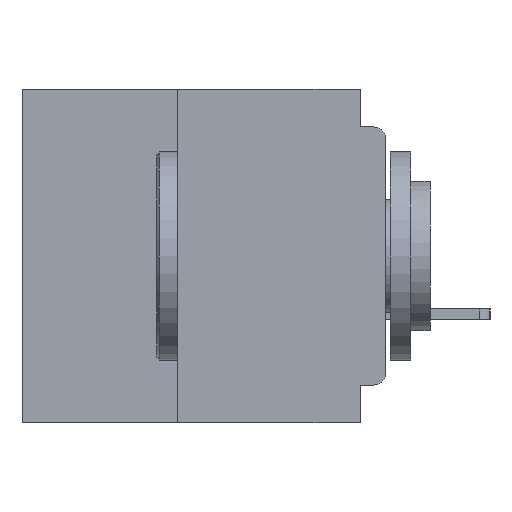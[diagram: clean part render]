
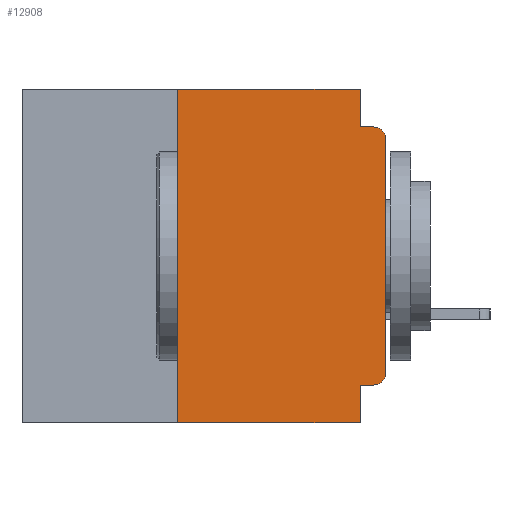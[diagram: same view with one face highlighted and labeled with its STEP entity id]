
A CAD part, left-side view. The second image highlights one B-rep face of the part: STEP entity #12908.
In plain terms, the highlighted planar face has unit normal (-1, 0, 0).
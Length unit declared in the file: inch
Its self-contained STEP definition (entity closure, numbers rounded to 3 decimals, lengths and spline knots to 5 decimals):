
#207 = LINE ( 'NONE', #11736, #41279 ) ;
#290 = VECTOR ( 'NONE', #2912, 39.37008 ) ;
#741 = VERTEX_POINT ( 'NONE', #13909 ) ;
#750 = DIRECTION ( 'NONE',  ( 0., 0., -1. ) ) ;
#1544 = LINE ( 'NONE', #10858, #290 ) ;
#1704 = EDGE_CURVE ( 'NONE', #27316, #12197, #5663, .T. ) ;
#1719 = ORIENTED_EDGE ( 'NONE', *, *, #18639, .F. ) ;
#1902 = VERTEX_POINT ( 'NONE', #48095 ) ;
#2888 = VERTEX_POINT ( 'NONE', #45726 ) ;
#2912 = DIRECTION ( 'NONE',  ( 0., 1., 0. ) ) ;
#3446 = LINE ( 'NONE', #10062, #22133 ) ;
#4412 = VECTOR ( 'NONE', #18042, 39.37008 ) ;
#4454 = EDGE_CURVE ( 'NONE', #5915, #27316, #51467, .T. ) ;
#4998 = DIRECTION ( 'NONE',  ( 0., 0., -1. ) ) ;
#5009 = CARTESIAN_POINT ( 'NONE',  ( 0., 0.437, -0.4 ) ) ;
#5066 = DIRECTION ( 'NONE',  ( -1., 0., 0. ) ) ;
#5075 = CARTESIAN_POINT ( 'NONE',  ( 0., 0.015, -0.34 ) ) ;
#5244 = PLANE ( 'NONE',  #33395 ) ;
#5475 = ORIENTED_EDGE ( 'NONE', *, *, #14504, .F. ) ;
#5663 = LINE ( 'NONE', #18956, #4412 ) ;
#5915 = VERTEX_POINT ( 'NONE', #47709 ) ;
#6281 = DIRECTION ( 'NONE',  ( 0., -1., 0. ) ) ;
#6307 = VECTOR ( 'NONE', #750, 39.37008 ) ;
#6487 = VERTEX_POINT ( 'NONE', #47653 ) ;
#6509 = DIRECTION ( 'NONE',  ( 0., -1., 0. ) ) ;
#9202 = DIRECTION ( 'NONE',  ( 0., 0., -1. ) ) ;
#10062 = CARTESIAN_POINT ( 'NONE',  ( 0., 0., -0.045 ) ) ;
#10858 = CARTESIAN_POINT ( 'NONE',  ( 0., 0., -0.355 ) ) ;
#11176 = CARTESIAN_POINT ( 'NONE',  ( 0., 0.015, -0.06 ) ) ;
#11736 = CARTESIAN_POINT ( 'NONE',  ( 0., 0.031, 0. ) ) ;
#12105 = EDGE_CURVE ( 'NONE', #12197, #18398, #21471, .T. ) ;
#12197 = VERTEX_POINT ( 'NONE', #19746 ) ;
#12536 = CARTESIAN_POINT ( 'NONE',  ( 0., 0.015, -0.045 ) ) ;
#12908 = ADVANCED_FACE ( 'NONE', ( #34014 ), #5244, .F. ) ;
#13524 = ORIENTED_EDGE ( 'NONE', *, *, #14053, .F. ) ;
#13909 = CARTESIAN_POINT ( 'NONE',  ( 0., 0.031, -0.4 ) ) ;
#14053 = EDGE_CURVE ( 'NONE', #14677, #2888, #207, .T. ) ;
#14504 = EDGE_CURVE ( 'NONE', #43937, #14677, #30729, .T. ) ;
#14677 = VERTEX_POINT ( 'NONE', #43330 ) ;
#15201 = DIRECTION ( 'NONE',  ( 0., 0., -1. ) ) ;
#15613 = LINE ( 'NONE', #24624, #6307 ) ;
#17323 = ORIENTED_EDGE ( 'NONE', *, *, #47789, .T. ) ;
#18042 = DIRECTION ( 'NONE',  ( 0., 0., 1. ) ) ;
#18398 = VERTEX_POINT ( 'NONE', #12536 ) ;
#18639 = EDGE_CURVE ( 'NONE', #2888, #18398, #3446, .T. ) ;
#18956 = CARTESIAN_POINT ( 'NONE',  ( 0., 0., 0. ) ) ;
#19148 = ORIENTED_EDGE ( 'NONE', *, *, #1704, .T. ) ;
#19537 = EDGE_CURVE ( 'NONE', #5915, #6487, #1544, .T. ) ;
#19746 = CARTESIAN_POINT ( 'NONE',  ( 0., 0., -0.06 ) ) ;
#20414 = ORIENTED_EDGE ( 'NONE', *, *, #12105, .T. ) ;
#21067 = ORIENTED_EDGE ( 'NONE', *, *, #21550, .F. ) ;
#21471 = CIRCLE ( 'NONE', #25657, 0.015 ) ;
#21550 = EDGE_CURVE ( 'NONE', #6487, #741, #15613, .T. ) ;
#22133 = VECTOR ( 'NONE', #6281, 39.37008 ) ;
#24624 = CARTESIAN_POINT ( 'NONE',  ( 0., 0.031, -0.4 ) ) ;
#25094 = CARTESIAN_POINT ( 'NONE',  ( 0., 0.437, 0. ) ) ;
#25657 = AXIS2_PLACEMENT_3D ( 'NONE', #11176, #39026, #15201 ) ;
#26280 = EDGE_CURVE ( 'NONE', #1902, #43937, #48720, .T. ) ;
#26677 = ORIENTED_EDGE ( 'NONE', *, *, #26280, .F. ) ;
#27163 = DIRECTION ( 'NONE',  ( 0., 0., 1. ) ) ;
#27316 = VERTEX_POINT ( 'NONE', #47608 ) ;
#28867 = VECTOR ( 'NONE', #27163, 39.37008 ) ;
#29073 = DIRECTION ( 'NONE',  ( 0., -1., 0. ) ) ;
#30242 = LINE ( 'NONE', #5009, #39509 ) ;
#30729 = LINE ( 'NONE', #34370, #39993 ) ;
#31377 = AXIS2_PLACEMENT_3D ( 'NONE', #5075, #5066, #4998 ) ;
#31668 = ORIENTED_EDGE ( 'NONE', *, *, #19537, .F. ) ;
#32961 = EDGE_LOOP ( 'NONE', ( #19148, #20414, #1719, #13524, #5475, #26677, #17323, #21067, #31668, #43417 ) ) ;
#33128 = DIRECTION ( 'NONE',  ( 1., 0., 0. ) ) ;
#33395 = AXIS2_PLACEMENT_3D ( 'NONE', #25094, #33128, #9202 ) ;
#34014 = FACE_OUTER_BOUND ( 'NONE', #32961, .T. ) ;
#34370 = CARTESIAN_POINT ( 'NONE',  ( 0., 0.437, 0. ) ) ;
#39026 = DIRECTION ( 'NONE',  ( -1., 0., 0. ) ) ;
#39509 = VECTOR ( 'NONE', #29073, 39.37008 ) ;
#39575 = DIRECTION ( 'NONE',  ( 0., 0., -1. ) ) ;
#39993 = VECTOR ( 'NONE', #6509, 39.37008 ) ;
#41279 = VECTOR ( 'NONE', #39575, 39.37008 ) ;
#43330 = CARTESIAN_POINT ( 'NONE',  ( 0., 0.031, 0. ) ) ;
#43417 = ORIENTED_EDGE ( 'NONE', *, *, #4454, .T. ) ;
#43455 = CARTESIAN_POINT ( 'NONE',  ( 0., 0.25, 0. ) ) ;
#43937 = VERTEX_POINT ( 'NONE', #43455 ) ;
#45726 = CARTESIAN_POINT ( 'NONE',  ( 0., 0.031, -0.045 ) ) ;
#46910 = CARTESIAN_POINT ( 'NONE',  ( 0., 0.25, -0.4 ) ) ;
#47608 = CARTESIAN_POINT ( 'NONE',  ( 0., 0., -0.34 ) ) ;
#47653 = CARTESIAN_POINT ( 'NONE',  ( 0., 0.031, -0.355 ) ) ;
#47709 = CARTESIAN_POINT ( 'NONE',  ( 0., 0.015, -0.355 ) ) ;
#47789 = EDGE_CURVE ( 'NONE', #1902, #741, #30242, .T. ) ;
#48095 = CARTESIAN_POINT ( 'NONE',  ( 0., 0.25, -0.4 ) ) ;
#48720 = LINE ( 'NONE', #46910, #28867 ) ;
#51467 = CIRCLE ( 'NONE', #31377, 0.015 ) ;
